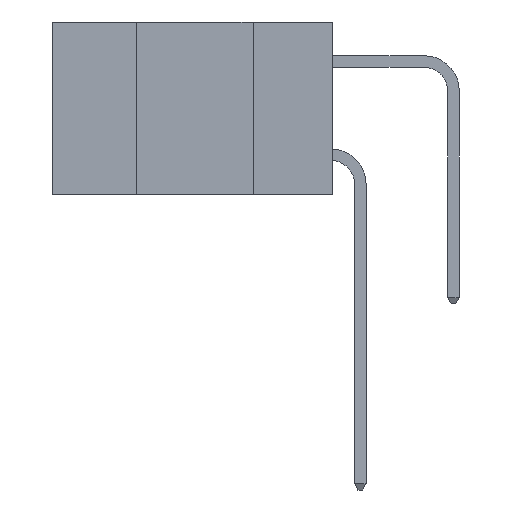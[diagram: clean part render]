
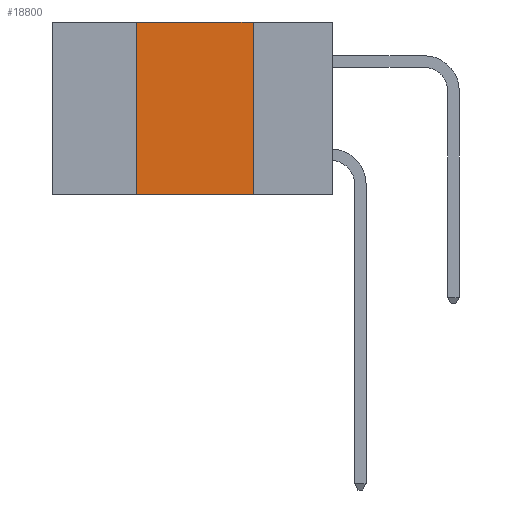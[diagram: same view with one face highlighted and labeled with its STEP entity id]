
A CAD part, left-side view. The second image highlights one B-rep face of the part: STEP entity #18800.
In plain terms, the highlighted planar face has unit normal (-1, 0, 0).
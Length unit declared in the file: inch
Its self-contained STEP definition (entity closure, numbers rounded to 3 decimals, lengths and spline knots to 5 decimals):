
#1843 = VERTEX_POINT ( 'NONE', #18819 ) ;
#2393 = CARTESIAN_POINT ( 'NONE',  ( 0., 0.6, 0. ) ) ;
#2484 = PLANE ( 'NONE',  #12502 ) ;
#2510 = VECTOR ( 'NONE', #13029, 39.37008 ) ;
#2686 = EDGE_CURVE ( 'NONE', #1843, #9260, #13696, .T. ) ;
#3391 = LINE ( 'NONE', #20205, #25601 ) ;
#4083 = EDGE_CURVE ( 'NONE', #19181, #9260, #5673, .T. ) ;
#4402 = EDGE_CURVE ( 'NONE', #14233, #19181, #3391, .T. ) ;
#4527 = CARTESIAN_POINT ( 'NONE',  ( 0., 0.17, -0.37 ) ) ;
#4603 = DIRECTION ( 'NONE',  ( 0., 0., -1. ) ) ;
#5673 = LINE ( 'NONE', #4527, #21730 ) ;
#5861 = ORIENTED_EDGE ( 'NONE', *, *, #4402, .F. ) ;
#6608 = DIRECTION ( 'NONE',  ( 0., 0., -1. ) ) ;
#8546 = ORIENTED_EDGE ( 'NONE', *, *, #8621, .F. ) ;
#8621 = EDGE_CURVE ( 'NONE', #1843, #14233, #17244, .T. ) ;
#9260 = VERTEX_POINT ( 'NONE', #25625 ) ;
#9522 = FACE_OUTER_BOUND ( 'NONE', #22995, .T. ) ;
#10930 = CARTESIAN_POINT ( 'NONE',  ( 0., 0.6, -0.37 ) ) ;
#11840 = CARTESIAN_POINT ( 'NONE',  ( 0., 0.17, 0. ) ) ;
#12502 = AXIS2_PLACEMENT_3D ( 'NONE', #2393, #17173, #4603 ) ;
#13029 = DIRECTION ( 'NONE',  ( 0., -1., 0. ) ) ;
#13696 = LINE ( 'NONE', #10930, #2510 ) ;
#14233 = VERTEX_POINT ( 'NONE', #19569 ) ;
#15145 = ORIENTED_EDGE ( 'NONE', *, *, #4083, .F. ) ;
#16091 = DIRECTION ( 'NONE',  ( 0., -1., 0. ) ) ;
#17173 = DIRECTION ( 'NONE',  ( 1., 0., 0. ) ) ;
#17244 = LINE ( 'NONE', #23474, #20833 ) ;
#18800 = ADVANCED_FACE ( 'NONE', ( #9522 ), #2484, .F. ) ;
#18819 = CARTESIAN_POINT ( 'NONE',  ( 0., 0.42, -0.37 ) ) ;
#19181 = VERTEX_POINT ( 'NONE', #11840 ) ;
#19569 = CARTESIAN_POINT ( 'NONE',  ( 0., 0.42, 0. ) ) ;
#20205 = CARTESIAN_POINT ( 'NONE',  ( 0., 0.6, 0. ) ) ;
#20833 = VECTOR ( 'NONE', #25554, 39.37008 ) ;
#21730 = VECTOR ( 'NONE', #6608, 39.37008 ) ;
#22995 = EDGE_LOOP ( 'NONE', ( #15145, #5861, #8546, #23204 ) ) ;
#23204 = ORIENTED_EDGE ( 'NONE', *, *, #2686, .T. ) ;
#23474 = CARTESIAN_POINT ( 'NONE',  ( 0., 0.42, -0.37 ) ) ;
#25554 = DIRECTION ( 'NONE',  ( 0., 0., 1. ) ) ;
#25601 = VECTOR ( 'NONE', #16091, 39.37008 ) ;
#25625 = CARTESIAN_POINT ( 'NONE',  ( 0., 0.17, -0.37 ) ) ;
